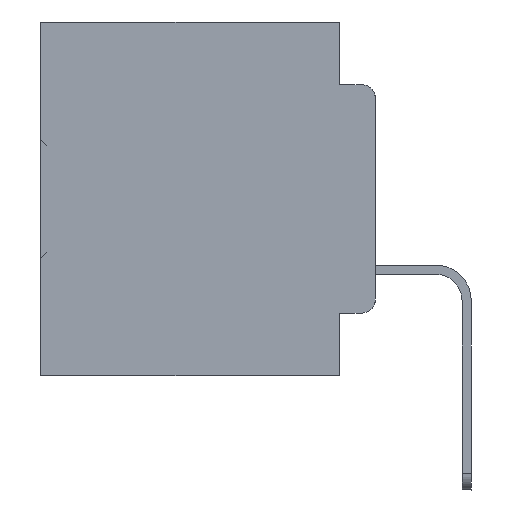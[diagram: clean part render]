
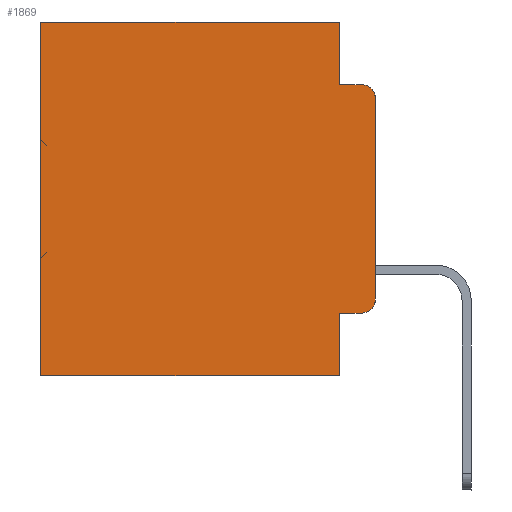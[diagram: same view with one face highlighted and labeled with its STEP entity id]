
A CAD part, left-side view. The second image highlights one B-rep face of the part: STEP entity #1869.
In plain terms, the highlighted planar face has unit normal (-1, 0, 0).
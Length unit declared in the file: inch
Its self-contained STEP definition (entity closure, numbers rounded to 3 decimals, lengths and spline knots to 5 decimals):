
#464 = CARTESIAN_POINT ( 'NONE',  ( 0.298, 0., 0. ) ) ;
#746 = ORIENTED_EDGE ( 'NONE', *, *, #35873, .T. ) ;
#1869 = ADVANCED_FACE ( 'NONE', ( #29284 ), #3610, .F. ) ;
#2150 = EDGE_CURVE ( 'NONE', #28621, #3903, #9942, .T. ) ;
#3145 = ORIENTED_EDGE ( 'NONE', *, *, #19107, .F. ) ;
#3156 = VERTEX_POINT ( 'NONE', #12434 ) ;
#3309 = AXIS2_PLACEMENT_3D ( 'NONE', #13288, #24937, #33257 ) ;
#3610 = PLANE ( 'NONE',  #18510 ) ;
#3696 = EDGE_CURVE ( 'NONE', #25977, #4723, #17095, .T. ) ;
#3903 = VERTEX_POINT ( 'NONE', #28375 ) ;
#4117 = ORIENTED_EDGE ( 'NONE', *, *, #21934, .F. ) ;
#4723 = VERTEX_POINT ( 'NONE', #6951 ) ;
#5001 = CARTESIAN_POINT ( 'NONE',  ( 0.298, 0.051, 0. ) ) ;
#5089 = ORIENTED_EDGE ( 'NONE', *, *, #2150, .T. ) ;
#5859 = LINE ( 'NONE', #24505, #36871 ) ;
#6652 = CARTESIAN_POINT ( 'NONE',  ( 0.298, 0.473, 0. ) ) ;
#6943 = CARTESIAN_POINT ( 'NONE',  ( 0.298, 0., 0. ) ) ;
#6951 = CARTESIAN_POINT ( 'NONE',  ( 0.298, 0., -0.3915 ) ) ;
#7682 = DIRECTION ( 'NONE',  ( 0., 0., -1. ) ) ;
#8317 = LINE ( 'NONE', #28866, #22741 ) ;
#8816 = LINE ( 'NONE', #6652, #23230 ) ;
#9298 = DIRECTION ( 'NONE',  ( 0., 0., -1. ) ) ;
#9358 = CARTESIAN_POINT ( 'NONE',  ( 0.298, 0.02, -0.3915 ) ) ;
#9600 = CARTESIAN_POINT ( 'NONE',  ( 0.298, 0.051, 0. ) ) ;
#9611 = ORIENTED_EDGE ( 'NONE', *, *, #14237, .T. ) ;
#9672 = CARTESIAN_POINT ( 'NONE',  ( 0.298, 0.02, -0.4115 ) ) ;
#9942 = CIRCLE ( 'NONE', #3309, 0.02 ) ;
#10549 = VERTEX_POINT ( 'NONE', #19562 ) ;
#10565 = CARTESIAN_POINT ( 'NONE',  ( 0.298, 0., 0. ) ) ;
#10830 = DIRECTION ( 'NONE',  ( 0., 0., -1. ) ) ;
#12434 = CARTESIAN_POINT ( 'NONE',  ( 0.298, 0.473, -0.5 ) ) ;
#12534 = EDGE_CURVE ( 'NONE', #28621, #4723, #34842, .T. ) ;
#12544 = DIRECTION ( 'NONE',  ( 0., 0., -1. ) ) ;
#13021 = AXIS2_PLACEMENT_3D ( 'NONE', #9358, #32369, #13346 ) ;
#13288 = CARTESIAN_POINT ( 'NONE',  ( 0.298, 0.02, -0.1085 ) ) ;
#13346 = DIRECTION ( 'NONE',  ( 0., 0., -1. ) ) ;
#14237 = EDGE_CURVE ( 'NONE', #34602, #18691, #34280, .T. ) ;
#15223 = ORIENTED_EDGE ( 'NONE', *, *, #20074, .T. ) ;
#16080 = LINE ( 'NONE', #29249, #19684 ) ;
#16224 = EDGE_LOOP ( 'NONE', ( #36405, #5089, #29634, #16651, #9611, #746, #4117, #3145, #15223, #34745 ) ) ;
#16651 = ORIENTED_EDGE ( 'NONE', *, *, #17898, .F. ) ;
#17095 = CIRCLE ( 'NONE', #13021, 0.02 ) ;
#17555 = VERTEX_POINT ( 'NONE', #20690 ) ;
#17693 = CARTESIAN_POINT ( 'NONE',  ( 0.298, 0.051, 0. ) ) ;
#17898 = EDGE_CURVE ( 'NONE', #34602, #17555, #28591, .T. ) ;
#18510 = AXIS2_PLACEMENT_3D ( 'NONE', #464, #31929, #9298 ) ;
#18691 = VERTEX_POINT ( 'NONE', #30860 ) ;
#19107 = EDGE_CURVE ( 'NONE', #34625, #10549, #27379, .T. ) ;
#19562 = CARTESIAN_POINT ( 'NONE',  ( 0.298, 0.051, -0.5 ) ) ;
#19684 = VECTOR ( 'NONE', #37313, 39.37008 ) ;
#20074 = EDGE_CURVE ( 'NONE', #34625, #25977, #16080, .T. ) ;
#20690 = CARTESIAN_POINT ( 'NONE',  ( 0.298, 0.051, -0.0885 ) ) ;
#21889 = VECTOR ( 'NONE', #10830, 39.37008 ) ;
#21934 = EDGE_CURVE ( 'NONE', #10549, #3156, #8317, .T. ) ;
#22741 = VECTOR ( 'NONE', #37294, 39.37008 ) ;
#23230 = VECTOR ( 'NONE', #37222, 39.37008 ) ;
#23928 = DIRECTION ( 'NONE',  ( 0., 1., 0. ) ) ;
#24280 = EDGE_CURVE ( 'NONE', #17555, #3903, #5859, .T. ) ;
#24505 = CARTESIAN_POINT ( 'NONE',  ( 0.298, 0.051, -0.0885 ) ) ;
#24937 = DIRECTION ( 'NONE',  ( -1., 0., 0. ) ) ;
#25977 = VERTEX_POINT ( 'NONE', #9672 ) ;
#27379 = LINE ( 'NONE', #9600, #28252 ) ;
#28252 = VECTOR ( 'NONE', #12544, 39.37008 ) ;
#28375 = CARTESIAN_POINT ( 'NONE',  ( 0.298, 0.02, -0.0885 ) ) ;
#28591 = LINE ( 'NONE', #5001, #21889 ) ;
#28621 = VERTEX_POINT ( 'NONE', #31201 ) ;
#28866 = CARTESIAN_POINT ( 'NONE',  ( 0.298, 0., -0.5 ) ) ;
#29249 = CARTESIAN_POINT ( 'NONE',  ( 0.298, 0.051, -0.4115 ) ) ;
#29284 = FACE_OUTER_BOUND ( 'NONE', #16224, .T. ) ;
#29564 = CARTESIAN_POINT ( 'NONE',  ( 0.298, 0.051, -0.4115 ) ) ;
#29634 = ORIENTED_EDGE ( 'NONE', *, *, #24280, .F. ) ;
#30860 = CARTESIAN_POINT ( 'NONE',  ( 0.298, 0.473, 0. ) ) ;
#31201 = CARTESIAN_POINT ( 'NONE',  ( 0.298, 0., -0.1085 ) ) ;
#31929 = DIRECTION ( 'NONE',  ( 1., 0., 0. ) ) ;
#32369 = DIRECTION ( 'NONE',  ( -1., 0., 0. ) ) ;
#33257 = DIRECTION ( 'NONE',  ( 0., 0., -1. ) ) ;
#33396 = VECTOR ( 'NONE', #23928, 39.37008 ) ;
#34280 = LINE ( 'NONE', #6943, #33396 ) ;
#34602 = VERTEX_POINT ( 'NONE', #17693 ) ;
#34625 = VERTEX_POINT ( 'NONE', #29564 ) ;
#34745 = ORIENTED_EDGE ( 'NONE', *, *, #3696, .T. ) ;
#34842 = LINE ( 'NONE', #10565, #35737 ) ;
#35737 = VECTOR ( 'NONE', #7682, 39.37008 ) ;
#35873 = EDGE_CURVE ( 'NONE', #18691, #3156, #8816, .T. ) ;
#36039 = DIRECTION ( 'NONE',  ( 0., -1., 0. ) ) ;
#36405 = ORIENTED_EDGE ( 'NONE', *, *, #12534, .F. ) ;
#36871 = VECTOR ( 'NONE', #36039, 39.37008 ) ;
#37222 = DIRECTION ( 'NONE',  ( 0., 0., -1. ) ) ;
#37294 = DIRECTION ( 'NONE',  ( 0., 1., 0. ) ) ;
#37313 = DIRECTION ( 'NONE',  ( 0., -1., 0. ) ) ;
